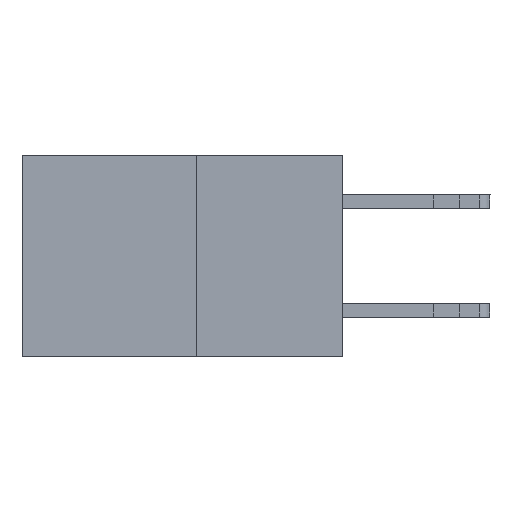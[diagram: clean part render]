
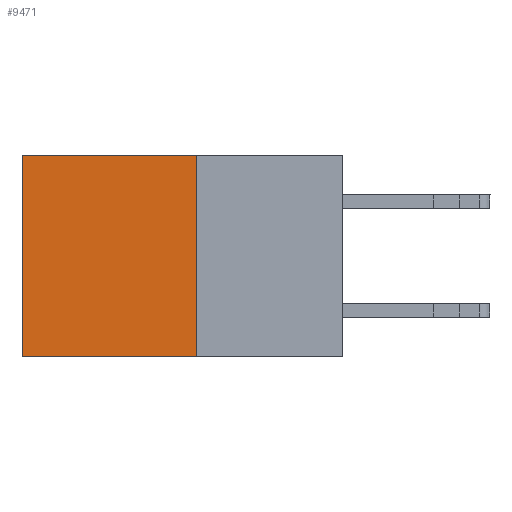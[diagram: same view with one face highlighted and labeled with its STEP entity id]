
A CAD part, left-side view. The second image highlights one B-rep face of the part: STEP entity #9471.
In plain terms, the highlighted planar face has unit normal (-1, 0, 0).
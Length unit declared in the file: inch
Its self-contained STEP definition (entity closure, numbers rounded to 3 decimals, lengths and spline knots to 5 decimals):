
#337 = EDGE_CURVE ( 'NONE', #9307, #6560, #14453, .T. ) ;
#1117 = VERTEX_POINT ( 'NONE', #9236 ) ;
#1970 = ORIENTED_EDGE ( 'NONE', *, *, #17565, .F. ) ;
#2365 = ORIENTED_EDGE ( 'NONE', *, *, #17000, .T. ) ;
#2813 = CARTESIAN_POINT ( 'NONE',  ( 0.277, 0.27, 0. ) ) ;
#3239 = DIRECTION ( 'NONE',  ( 0., 1., 0. ) ) ;
#3400 = DIRECTION ( 'NONE',  ( 1., 0., 0. ) ) ;
#3481 = VECTOR ( 'NONE', #3786, 39.37008 ) ;
#3786 = DIRECTION ( 'NONE',  ( 0., 1., 0. ) ) ;
#4256 = LINE ( 'NONE', #19203, #10681 ) ;
#4533 = LINE ( 'NONE', #18393, #17764 ) ;
#5731 = CARTESIAN_POINT ( 'NONE',  ( 0.277, 0.59, 0. ) ) ;
#5797 = CARTESIAN_POINT ( 'NONE',  ( 0.277, 0.59, -0.37 ) ) ;
#6309 = ORIENTED_EDGE ( 'NONE', *, *, #12391, .F. ) ;
#6560 = VERTEX_POINT ( 'NONE', #5731 ) ;
#8640 = DIRECTION ( 'NONE',  ( 0., 0., -1. ) ) ;
#9236 = CARTESIAN_POINT ( 'NONE',  ( 0.277, 0.59, -0.37 ) ) ;
#9283 = DIRECTION ( 'NONE',  ( 0., 0., -1. ) ) ;
#9307 = VERTEX_POINT ( 'NONE', #2813 ) ;
#9471 = ADVANCED_FACE ( 'NONE', ( #12464 ), #10578, .F. ) ;
#10578 = PLANE ( 'NONE',  #19377 ) ;
#10681 = VECTOR ( 'NONE', #8640, 39.37008 ) ;
#11791 = VERTEX_POINT ( 'NONE', #14542 ) ;
#12391 = EDGE_CURVE ( 'NONE', #9307, #11791, #4256, .T. ) ;
#12464 = FACE_OUTER_BOUND ( 'NONE', #15346, .T. ) ;
#14453 = LINE ( 'NONE', #19239, #3481 ) ;
#14542 = CARTESIAN_POINT ( 'NONE',  ( 0.277, 0.27, -0.37 ) ) ;
#14574 = ORIENTED_EDGE ( 'NONE', *, *, #337, .T. ) ;
#15346 = EDGE_LOOP ( 'NONE', ( #2365, #1970, #6309, #14574 ) ) ;
#15366 = DIRECTION ( 'NONE',  ( 0., 0., -1. ) ) ;
#17000 = EDGE_CURVE ( 'NONE', #6560, #1117, #19450, .T. ) ;
#17070 = CARTESIAN_POINT ( 'NONE',  ( 0.277, 0.27, -0.37 ) ) ;
#17565 = EDGE_CURVE ( 'NONE', #11791, #1117, #4533, .T. ) ;
#17764 = VECTOR ( 'NONE', #3239, 39.37008 ) ;
#18393 = CARTESIAN_POINT ( 'NONE',  ( 0.277, 0.27, -0.37 ) ) ;
#19203 = CARTESIAN_POINT ( 'NONE',  ( 0.277, 0.27, -0.37 ) ) ;
#19239 = CARTESIAN_POINT ( 'NONE',  ( 0.277, 0.27, 0. ) ) ;
#19377 = AXIS2_PLACEMENT_3D ( 'NONE', #17070, #3400, #9283 ) ;
#19423 = VECTOR ( 'NONE', #15366, 39.37008 ) ;
#19450 = LINE ( 'NONE', #5797, #19423 ) ;
